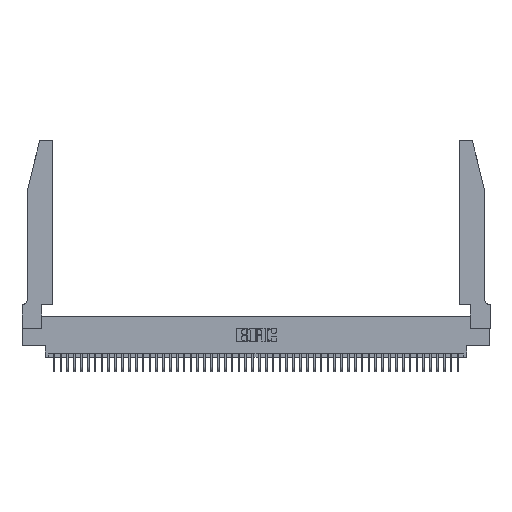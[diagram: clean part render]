
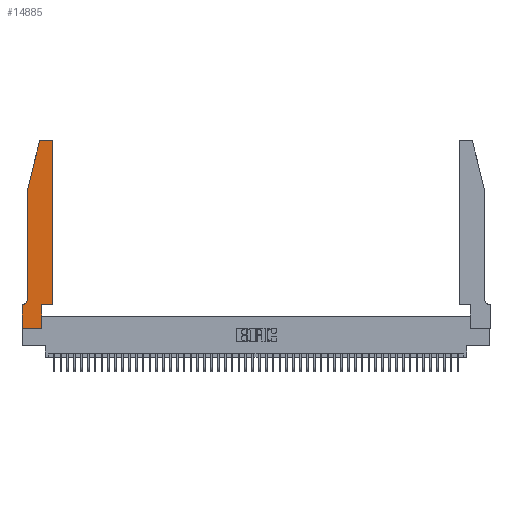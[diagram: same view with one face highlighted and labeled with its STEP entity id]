
A CAD part, top view. The second image highlights one B-rep face of the part: STEP entity #14885.
In plain terms, the highlighted planar face has unit normal (0, 0, 1).
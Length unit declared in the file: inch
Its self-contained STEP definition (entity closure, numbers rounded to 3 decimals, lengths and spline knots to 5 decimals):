
#811 = VERTEX_POINT ( 'NONE', #31352 ) ;
#1640 = CARTESIAN_POINT ( 'NONE',  ( 0.4505, 0.35, 0.37 ) ) ;
#3353 = EDGE_CURVE ( 'NONE', #44001, #21940, #25701, .T. ) ;
#3921 = EDGE_CURVE ( 'NONE', #30405, #20157, #10183, .T. ) ;
#4016 = LINE ( 'NONE', #49884, #44842 ) ;
#4432 = CARTESIAN_POINT ( 'NONE',  ( 0.4505, 2.72, 0.37 ) ) ;
#6007 = CARTESIAN_POINT ( 'NONE',  ( 0.2865, 0.35, 0.37 ) ) ;
#6272 = VERTEX_POINT ( 'NONE', #33571 ) ;
#7056 = EDGE_CURVE ( 'NONE', #6272, #23211, #40844, .T. ) ;
#7579 = ORIENTED_EDGE ( 'NONE', *, *, #37973, .T. ) ;
#8312 = CARTESIAN_POINT ( 'NONE',  ( 0., 0., 0.37 ) ) ;
#8547 = CARTESIAN_POINT ( 'NONE',  ( 0.0755, 2., 0.37 ) ) ;
#8660 = DIRECTION ( 'NONE',  ( 1., 0., 0. ) ) ;
#9070 = ORIENTED_EDGE ( 'NONE', *, *, #3353, .T. ) ;
#9571 = CARTESIAN_POINT ( 'NONE',  ( 0., 0.35, 0.37 ) ) ;
#9729 = DIRECTION ( 'NONE',  ( 0., 0., 1. ) ) ;
#10050 = DIRECTION ( 'NONE',  ( 0., 1., 0. ) ) ;
#10183 = LINE ( 'NONE', #36437, #29937 ) ;
#10761 = LINE ( 'NONE', #30839, #20053 ) ;
#11166 = CARTESIAN_POINT ( 'NONE',  ( 0.2865, 0.35, 0.37 ) ) ;
#11532 = EDGE_CURVE ( 'NONE', #811, #44001, #10761, .T. ) ;
#12516 = VECTOR ( 'NONE', #30738, 39.37008 ) ;
#12798 = ORIENTED_EDGE ( 'NONE', *, *, #29715, .T. ) ;
#12897 = VECTOR ( 'NONE', #16452, 39.37008 ) ;
#13271 = AXIS2_PLACEMENT_3D ( 'NONE', #46199, #22669, #50094 ) ;
#13612 = DIRECTION ( 'NONE',  ( 1., 0., 0. ) ) ;
#14885 = ADVANCED_FACE ( 'NONE', ( #22984 ), #29244, .T. ) ;
#15215 = VECTOR ( 'NONE', #43494, 39.37008 ) ;
#15779 = CARTESIAN_POINT ( 'NONE',  ( 0.0755, 0.35, 0.37 ) ) ;
#16273 = CARTESIAN_POINT ( 'NONE',  ( 0.2865, 0., 0.37 ) ) ;
#16452 = DIRECTION ( 'NONE',  ( -0.239, -0.971, 0. ) ) ;
#16723 = CARTESIAN_POINT ( 'NONE',  ( 0.4205, 2.72, 0.37 ) ) ;
#17013 = CARTESIAN_POINT ( 'NONE',  ( 0.0055, 0.35, 0.37 ) ) ;
#18247 = ORIENTED_EDGE ( 'NONE', *, *, #24041, .T. ) ;
#18469 = VERTEX_POINT ( 'NONE', #46459 ) ;
#19183 = DIRECTION ( 'NONE',  ( -1., 0., 0. ) ) ;
#19911 = VERTEX_POINT ( 'NONE', #43264 ) ;
#20053 = VECTOR ( 'NONE', #19183, 39.37008 ) ;
#20157 = VERTEX_POINT ( 'NONE', #1640 ) ;
#20579 = EDGE_CURVE ( 'NONE', #50575, #48955, #44164, .T. ) ;
#20675 = DIRECTION ( 'NONE',  ( 1., 0., 0. ) ) ;
#21733 = EDGE_LOOP ( 'NONE', ( #47590, #9070, #41872, #51003, #47364, #7579, #18247, #28782, #43380, #48924, #12798, #34277 ) ) ;
#21940 = VERTEX_POINT ( 'NONE', #29487 ) ;
#22031 = VECTOR ( 'NONE', #8660, 39.37008 ) ;
#22282 = CIRCLE ( 'NONE', #37630, 0.03 ) ;
#22669 = DIRECTION ( 'NONE',  ( 0., 0., -1. ) ) ;
#22984 = FACE_OUTER_BOUND ( 'NONE', #21733, .T. ) ;
#23211 = VERTEX_POINT ( 'NONE', #17013 ) ;
#24041 = EDGE_CURVE ( 'NONE', #19911, #50575, #43886, .T. ) ;
#25701 = CIRCLE ( 'NONE', #47741, 0.03 ) ;
#26771 = CARTESIAN_POINT ( 'NONE',  ( 0., 0., 0.37 ) ) ;
#26901 = LINE ( 'NONE', #6007, #34907 ) ;
#28782 = ORIENTED_EDGE ( 'NONE', *, *, #20579, .T. ) ;
#29244 = PLANE ( 'NONE',  #42542 ) ;
#29487 = CARTESIAN_POINT ( 'NONE',  ( 0.25487, 2.72718, 0.37 ) ) ;
#29715 = EDGE_CURVE ( 'NONE', #20157, #44865, #4016, .T. ) ;
#29937 = VECTOR ( 'NONE', #40398, 39.37008 ) ;
#30405 = VERTEX_POINT ( 'NONE', #11166 ) ;
#30738 = DIRECTION ( 'NONE',  ( 0., -1., 0. ) ) ;
#30839 = CARTESIAN_POINT ( 'NONE',  ( 0.2605, 2.75, 0.37 ) ) ;
#30904 = EDGE_CURVE ( 'NONE', #48955, #30405, #26901, .T. ) ;
#31352 = CARTESIAN_POINT ( 'NONE',  ( 0.4205, 2.75, 0.37 ) ) ;
#33377 = CARTESIAN_POINT ( 'NONE',  ( 0.284, 2.72, 0.37 ) ) ;
#33571 = CARTESIAN_POINT ( 'NONE',  ( 0.0755, 0.42, 0.37 ) ) ;
#34277 = ORIENTED_EDGE ( 'NONE', *, *, #47697, .T. ) ;
#34321 = DIRECTION ( 'NONE',  ( 0., 1., 0. ) ) ;
#34907 = VECTOR ( 'NONE', #10050, 39.37008 ) ;
#36112 = LINE ( 'NONE', #39571, #15215 ) ;
#36437 = CARTESIAN_POINT ( 'NONE',  ( 0.4505, 0.35, 0.37 ) ) ;
#37191 = DIRECTION ( 'NONE',  ( 0., 0., 1. ) ) ;
#37338 = DIRECTION ( 'NONE',  ( 1., 0., 0. ) ) ;
#37630 = AXIS2_PLACEMENT_3D ( 'NONE', #16723, #44200, #20675 ) ;
#37883 = VECTOR ( 'NONE', #43271, 39.37008 ) ;
#37973 = EDGE_CURVE ( 'NONE', #23211, #19911, #47074, .T. ) ;
#39571 = CARTESIAN_POINT ( 'NONE',  ( 0.0755, 2., 0.37 ) ) ;
#40294 = CARTESIAN_POINT ( 'NONE',  ( 0., 0., 0.37 ) ) ;
#40398 = DIRECTION ( 'NONE',  ( 1., 0., 0. ) ) ;
#40844 = CIRCLE ( 'NONE', #13271, 0.07 ) ;
#41872 = ORIENTED_EDGE ( 'NONE', *, *, #49011, .T. ) ;
#42443 = EDGE_CURVE ( 'NONE', #18469, #6272, #36112, .T. ) ;
#42542 = AXIS2_PLACEMENT_3D ( 'NONE', #9571, #37191, #13612 ) ;
#43264 = CARTESIAN_POINT ( 'NONE',  ( 0., 0.35, 0.37 ) ) ;
#43271 = DIRECTION ( 'NONE',  ( -1., 0., 0. ) ) ;
#43380 = ORIENTED_EDGE ( 'NONE', *, *, #30904, .T. ) ;
#43494 = DIRECTION ( 'NONE',  ( 0., -1., 0. ) ) ;
#43886 = LINE ( 'NONE', #26771, #12516 ) ;
#44001 = VERTEX_POINT ( 'NONE', #45552 ) ;
#44164 = LINE ( 'NONE', #40294, #22031 ) ;
#44200 = DIRECTION ( 'NONE',  ( 0., 0., 1. ) ) ;
#44276 = LINE ( 'NONE', #8547, #12897 ) ;
#44842 = VECTOR ( 'NONE', #34321, 39.37008 ) ;
#44865 = VERTEX_POINT ( 'NONE', #4432 ) ;
#45552 = CARTESIAN_POINT ( 'NONE',  ( 0.284, 2.75, 0.37 ) ) ;
#46199 = CARTESIAN_POINT ( 'NONE',  ( 0.0055, 0.42, 0.37 ) ) ;
#46459 = CARTESIAN_POINT ( 'NONE',  ( 0.0755, 2., 0.37 ) ) ;
#47074 = LINE ( 'NONE', #15779, #37883 ) ;
#47364 = ORIENTED_EDGE ( 'NONE', *, *, #7056, .T. ) ;
#47590 = ORIENTED_EDGE ( 'NONE', *, *, #11532, .T. ) ;
#47697 = EDGE_CURVE ( 'NONE', #44865, #811, #22282, .T. ) ;
#47741 = AXIS2_PLACEMENT_3D ( 'NONE', #33377, #9729, #37338 ) ;
#48924 = ORIENTED_EDGE ( 'NONE', *, *, #3921, .T. ) ;
#48955 = VERTEX_POINT ( 'NONE', #16273 ) ;
#49011 = EDGE_CURVE ( 'NONE', #21940, #18469, #44276, .T. ) ;
#49884 = CARTESIAN_POINT ( 'NONE',  ( 0.4505, 0.35, 0.37 ) ) ;
#50094 = DIRECTION ( 'NONE',  ( -1., 0., 0. ) ) ;
#50575 = VERTEX_POINT ( 'NONE', #8312 ) ;
#51003 = ORIENTED_EDGE ( 'NONE', *, *, #42443, .T. ) ;
